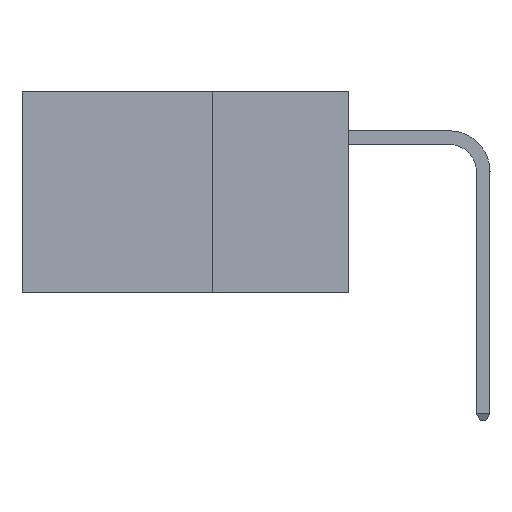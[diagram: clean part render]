
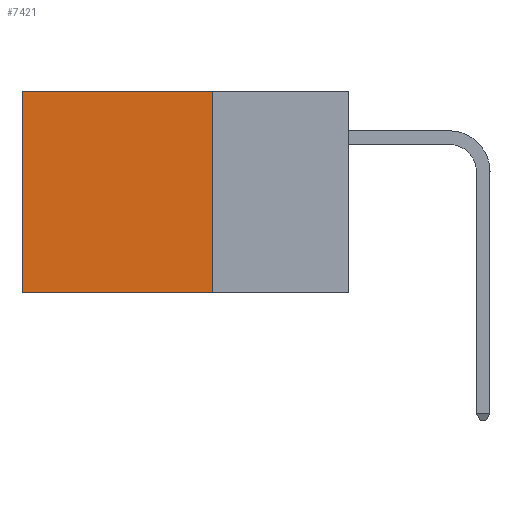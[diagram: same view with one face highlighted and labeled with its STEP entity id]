
A CAD part, left-side view. The second image highlights one B-rep face of the part: STEP entity #7421.
In plain terms, the highlighted planar face has unit normal (-1, 0, 0).
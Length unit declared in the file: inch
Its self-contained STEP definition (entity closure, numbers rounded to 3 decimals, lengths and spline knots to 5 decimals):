
#804 = VERTEX_POINT ( 'NONE', #8815 ) ;
#1140 = DIRECTION ( 'NONE',  ( 0., 0., -1. ) ) ;
#1443 = VECTOR ( 'NONE', #1140, 39.37008 ) ;
#1820 = VECTOR ( 'NONE', #8548, 39.37008 ) ;
#2143 = FACE_OUTER_BOUND ( 'NONE', #3061, .T. ) ;
#2297 = EDGE_CURVE ( 'NONE', #804, #7959, #5471, .T. ) ;
#2888 = VERTEX_POINT ( 'NONE', #3095 ) ;
#3061 = EDGE_LOOP ( 'NONE', ( #5328, #6754, #5929, #6217 ) ) ;
#3095 = CARTESIAN_POINT ( 'NONE',  ( 0.2875, 0.25, 0. ) ) ;
#3424 = LINE ( 'NONE', #4954, #1443 ) ;
#3441 = EDGE_CURVE ( 'NONE', #4361, #7959, #3424, .T. ) ;
#4361 = VERTEX_POINT ( 'NONE', #7995 ) ;
#4954 = CARTESIAN_POINT ( 'NONE',  ( 0.2875, 0.6, 0. ) ) ;
#5328 = ORIENTED_EDGE ( 'NONE', *, *, #3441, .T. ) ;
#5471 = LINE ( 'NONE', #8398, #1820 ) ;
#5613 = LINE ( 'NONE', #6339, #9444 ) ;
#5911 = AXIS2_PLACEMENT_3D ( 'NONE', #8759, #8817, #8805 ) ;
#5929 = ORIENTED_EDGE ( 'NONE', *, *, #6417, .F. ) ;
#5957 = EDGE_CURVE ( 'NONE', #2888, #4361, #5613, .T. ) ;
#6054 = DIRECTION ( 'NONE',  ( 0., 0., -1. ) ) ;
#6217 = ORIENTED_EDGE ( 'NONE', *, *, #5957, .T. ) ;
#6339 = CARTESIAN_POINT ( 'NONE',  ( 0.2875, 0.25, 0. ) ) ;
#6417 = EDGE_CURVE ( 'NONE', #2888, #804, #7282, .T. ) ;
#6754 = ORIENTED_EDGE ( 'NONE', *, *, #2297, .F. ) ;
#6841 = CARTESIAN_POINT ( 'NONE',  ( 0.2875, 0.25, 0. ) ) ;
#7064 = VECTOR ( 'NONE', #6054, 39.37008 ) ;
#7282 = LINE ( 'NONE', #6841, #7064 ) ;
#7421 = ADVANCED_FACE ( 'NONE', ( #2143 ), #8790, .F. ) ;
#7959 = VERTEX_POINT ( 'NONE', #8492 ) ;
#7995 = CARTESIAN_POINT ( 'NONE',  ( 0.2875, 0.6, 0. ) ) ;
#8038 = DIRECTION ( 'NONE',  ( 0., 1., 0. ) ) ;
#8398 = CARTESIAN_POINT ( 'NONE',  ( 0.2875, 0.25, -0.37 ) ) ;
#8492 = CARTESIAN_POINT ( 'NONE',  ( 0.2875, 0.6, -0.37 ) ) ;
#8548 = DIRECTION ( 'NONE',  ( 0., 1., 0. ) ) ;
#8759 = CARTESIAN_POINT ( 'NONE',  ( 0.2875, 0.25, 0. ) ) ;
#8790 = PLANE ( 'NONE',  #5911 ) ;
#8805 = DIRECTION ( 'NONE',  ( 0., 0., -1. ) ) ;
#8815 = CARTESIAN_POINT ( 'NONE',  ( 0.2875, 0.25, -0.37 ) ) ;
#8817 = DIRECTION ( 'NONE',  ( 1., 0., 0. ) ) ;
#9444 = VECTOR ( 'NONE', #8038, 39.37008 ) ;
